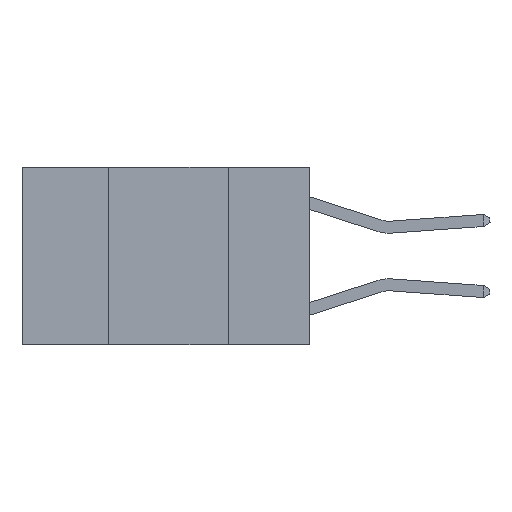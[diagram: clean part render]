
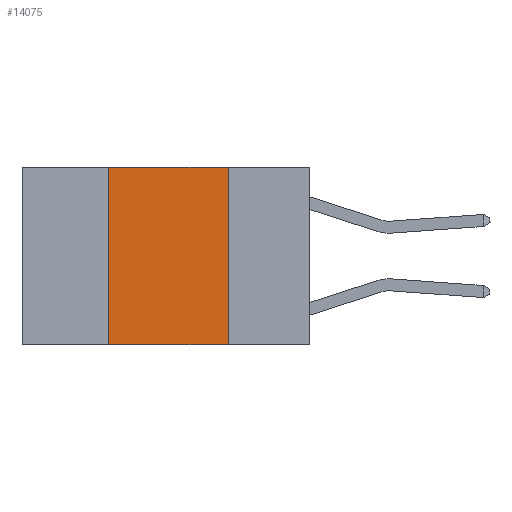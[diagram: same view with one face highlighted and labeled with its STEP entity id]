
A CAD part, left-side view. The second image highlights one B-rep face of the part: STEP entity #14075.
In plain terms, the highlighted planar face has unit normal (-1, 0, 0).
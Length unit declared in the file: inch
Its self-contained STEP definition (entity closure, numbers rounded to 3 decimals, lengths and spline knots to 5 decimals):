
#510 = CARTESIAN_POINT ( 'NONE',  ( 0., 0.42, -0.37 ) ) ;
#1468 = VERTEX_POINT ( 'NONE', #510 ) ;
#1697 = PLANE ( 'NONE',  #7264 ) ;
#1967 = FACE_OUTER_BOUND ( 'NONE', #20453, .T. ) ;
#2565 = LINE ( 'NONE', #10327, #3619 ) ;
#3619 = VECTOR ( 'NONE', #22201, 39.37008 ) ;
#4294 = VECTOR ( 'NONE', #16739, 39.37008 ) ;
#4531 = ORIENTED_EDGE ( 'NONE', *, *, #10798, .T. ) ;
#4750 = CARTESIAN_POINT ( 'NONE',  ( 0., 0.6, -0.37 ) ) ;
#4802 = ORIENTED_EDGE ( 'NONE', *, *, #5811, .F. ) ;
#5101 = EDGE_CURVE ( 'NONE', #6797, #17244, #20084, .T. ) ;
#5811 = EDGE_CURVE ( 'NONE', #1468, #9059, #8739, .T. ) ;
#6280 = DIRECTION ( 'NONE',  ( 0., 0., -1. ) ) ;
#6672 = ORIENTED_EDGE ( 'NONE', *, *, #5101, .F. ) ;
#6797 = VERTEX_POINT ( 'NONE', #14150 ) ;
#7264 = AXIS2_PLACEMENT_3D ( 'NONE', #12204, #13909, #20245 ) ;
#7725 = VECTOR ( 'NONE', #24672, 39.37008 ) ;
#8739 = LINE ( 'NONE', #22577, #4294 ) ;
#9059 = VERTEX_POINT ( 'NONE', #23888 ) ;
#10327 = CARTESIAN_POINT ( 'NONE',  ( 0., 0.6, 0. ) ) ;
#10798 = EDGE_CURVE ( 'NONE', #1468, #17244, #22814, .T. ) ;
#10931 = VECTOR ( 'NONE', #6280, 39.37008 ) ;
#12204 = CARTESIAN_POINT ( 'NONE',  ( 0., 0.6, 0. ) ) ;
#13909 = DIRECTION ( 'NONE',  ( 1., 0., 0. ) ) ;
#14075 = ADVANCED_FACE ( 'NONE', ( #1967 ), #1697, .F. ) ;
#14150 = CARTESIAN_POINT ( 'NONE',  ( 0., 0.17, 0. ) ) ;
#16739 = DIRECTION ( 'NONE',  ( 0., 0., 1. ) ) ;
#17244 = VERTEX_POINT ( 'NONE', #21776 ) ;
#20084 = LINE ( 'NONE', #22080, #10931 ) ;
#20245 = DIRECTION ( 'NONE',  ( 0., 0., -1. ) ) ;
#20453 = EDGE_LOOP ( 'NONE', ( #6672, #25084, #4802, #4531 ) ) ;
#21330 = EDGE_CURVE ( 'NONE', #9059, #6797, #2565, .T. ) ;
#21776 = CARTESIAN_POINT ( 'NONE',  ( 0., 0.17, -0.37 ) ) ;
#22080 = CARTESIAN_POINT ( 'NONE',  ( 0., 0.17, 0. ) ) ;
#22201 = DIRECTION ( 'NONE',  ( 0., -1., 0. ) ) ;
#22577 = CARTESIAN_POINT ( 'NONE',  ( 0., 0.42, 0. ) ) ;
#22814 = LINE ( 'NONE', #4750, #7725 ) ;
#23888 = CARTESIAN_POINT ( 'NONE',  ( 0., 0.42, 0. ) ) ;
#24672 = DIRECTION ( 'NONE',  ( 0., -1., 0. ) ) ;
#25084 = ORIENTED_EDGE ( 'NONE', *, *, #21330, .F. ) ;
